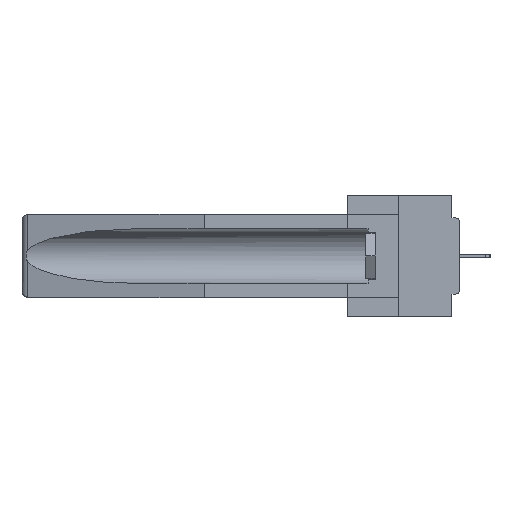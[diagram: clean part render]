
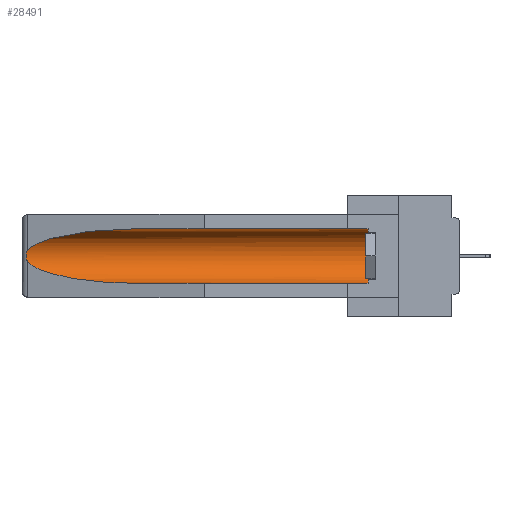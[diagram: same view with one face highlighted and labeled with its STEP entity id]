
A CAD part, left-side view. The second image highlights one B-rep face of the part: STEP entity #28491.
In plain terms, the highlighted cylindrical face has radius 2.857 mm (diameter 5.715 mm), a partial arc.
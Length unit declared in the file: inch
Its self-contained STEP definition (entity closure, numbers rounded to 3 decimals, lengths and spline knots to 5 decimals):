
#315 = CARTESIAN_POINT ( 'NONE',  ( 0.21114, 1.30732, -0.284 ) ) ;
#481 = LINE ( 'NONE', #18571, #19615 ) ;
#2081 = EDGE_CURVE ( 'NONE', #23746, #17120, #19596, .T. ) ;
#2356 = CARTESIAN_POINT ( 'NONE',  ( 0.26655, 1.53094, -0.18657 ) ) ;
#3650 = CARTESIAN_POINT ( 'NONE',  ( 0.155, 0.126, -0.059 ) ) ;
#4187 = ORIENTED_EDGE ( 'NONE', *, *, #26181, .T. ) ;
#4363 = CARTESIAN_POINT ( 'NONE',  ( 0.155, -0.30754, -0.059 ) ) ;
#4367 = LINE ( 'NONE', #4363, #23364 ) ;
#4866 = CARTESIAN_POINT ( 'NONE',  ( 0.26537, 1.52718, -0.19328 ) ) ;
#6810 = VERTEX_POINT ( 'NONE', #25696 ) ;
#7518 = CYLINDRICAL_SURFACE ( 'NONE', #13110, 0.1125 ) ;
#7524 = CARTESIAN_POINT ( 'NONE',  ( 0.155, 0.126, -0.1715 ) ) ;
#8186 = EDGE_CURVE ( 'NONE', #17120, #6810, #4367, .T. ) ;
#8830 = EDGE_CURVE ( 'NONE', #16722, #25071, #17514, .T. ) ;
#9365 = ORIENTED_EDGE ( 'NONE', *, *, #26984, .T. ) ;
#10338 = CARTESIAN_POINT ( 'NONE',  ( 0.26537, 1.52718, -0.19328 ) ) ;
#10518 = EDGE_CURVE ( 'NONE', #23746, #29125, #481, .T. ) ;
#10918 = ORIENTED_EDGE ( 'NONE', *, *, #10518, .F. ) ;
#11493 = CARTESIAN_POINT ( 'NONE',  ( 0.155, 1.07973, -0.059 ) ) ;
#12375 = CARTESIAN_POINT ( 'NONE',  ( 0.26537, 1.52718, -0.14972 ) ) ;
#13110 = AXIS2_PLACEMENT_3D ( 'NONE', #22780, #17799, #20341 ) ;
#13578 = DIRECTION ( 'NONE',  ( 0., 1., 0. ) ) ;
#13954 = CARTESIAN_POINT ( 'NONE',  ( 0.21114, 1.30732, -0.059 ) ) ;
#14334 = DIRECTION ( 'NONE',  ( 0., 1., 0. ) ) ;
#14829 = CARTESIAN_POINT ( 'NONE',  ( 0.2675, 1.53308, -0.16763 ) ) ;
#14921 = FACE_OUTER_BOUND ( 'NONE', #31670, .T. ) ;
#15785 = CARTESIAN_POINT ( 'NONE',  ( 0.26537, 1.52718, -0.19328 ) ) ;
#16444 = CARTESIAN_POINT ( 'NONE',  ( 0.26537, 1.52718, -0.14972 ) ) ;
#16722 = VERTEX_POINT ( 'NONE', #31481 ) ;
#17120 = VERTEX_POINT ( 'NONE', #3650 ) ;
#17335 = CARTESIAN_POINT ( 'NONE',  ( 0.2673, 1.53269, -0.17917 ) ) ;
#17514 = B_SPLINE_CURVE_WITH_KNOTS ( 'NONE', 3,
 ( #12375, #27003, #24555, #29465, #14829, #31859, #17335, #2356, #19803, #4866 ),
 .UNSPECIFIED., .F., .F.,
 ( 4, 2, 2, 2, 4 ),
 ( 0., 0.00029, 0.00058, 0.00087, 0.00117 ),
 .UNSPECIFIED. ) ;
#17539 = DIRECTION ( 'NONE',  ( 0., 0., 1. ) ) ;
#17799 = DIRECTION ( 'NONE',  ( 0., 1., 0. ) ) ;
#17816 = CARTESIAN_POINT ( 'NONE',  ( 0.155, 1.07973, -0.284 ) ) ;
#18571 = CARTESIAN_POINT ( 'NONE',  ( 0.155, -0.30754, -0.284 ) ) ;
#19596 = CIRCLE ( 'NONE', #26715, 0.1125 ) ;
#19615 = VECTOR ( 'NONE', #13578, 39.37008 ) ;
#19803 = CARTESIAN_POINT ( 'NONE',  ( 0.26597, 1.5296, -0.19026 ) ) ;
#20341 = DIRECTION ( 'NONE',  ( 0., 0., 1. ) ) ;
#20509 = CARTESIAN_POINT ( 'NONE',  ( 0.155, 1.07973, -0.284 ) ) ;
#22196 =( BOUNDED_CURVE ( )  B_SPLINE_CURVE ( 3, ( #11493, #13954, #31010, #16444 ),
 .UNSPECIFIED., .F., .F. ) 
 B_SPLINE_CURVE_WITH_KNOTS ( ( 4, 4 ),
 ( 4.71239, 6.08839 ),
 .UNSPECIFIED. ) 
 CURVE ( )  GEOMETRIC_REPRESENTATION_ITEM ( )  RATIONAL_B_SPLINE_CURVE ( ( 1., 0.848, 0.848, 1. ) ) 
 REPRESENTATION_ITEM ( '' )  );
#22448 = ORIENTED_EDGE ( 'NONE', *, *, #8830, .T. ) ;
#22780 = CARTESIAN_POINT ( 'NONE',  ( 0.155, -0.30754, -0.1715 ) ) ;
#23274 = CARTESIAN_POINT ( 'NONE',  ( 0.155, 0.126, -0.284 ) ) ;
#23364 = VECTOR ( 'NONE', #14334, 39.37008 ) ;
#23746 = VERTEX_POINT ( 'NONE', #23274 ) ;
#24555 = CARTESIAN_POINT ( 'NONE',  ( 0.26654, 1.53092, -0.15636 ) ) ;
#24713 = ORIENTED_EDGE ( 'NONE', *, *, #2081, .T. ) ;
#25071 = VERTEX_POINT ( 'NONE', #15785 ) ;
#25117 = DIRECTION ( 'NONE',  ( 0., -1., 0. ) ) ;
#25696 = CARTESIAN_POINT ( 'NONE',  ( 0.155, 1.07973, -0.059 ) ) ;
#26181 = EDGE_CURVE ( 'NONE', #25071, #29125, #31136, .T. ) ;
#26715 = AXIS2_PLACEMENT_3D ( 'NONE', #7524, #25117, #17539 ) ;
#26984 = EDGE_CURVE ( 'NONE', #6810, #16722, #22196, .T. ) ;
#27003 = CARTESIAN_POINT ( 'NONE',  ( 0.26597, 1.52961, -0.15275 ) ) ;
#28491 = ADVANCED_FACE ( 'NONE', ( #14921 ), #7518, .F. ) ;
#29125 = VERTEX_POINT ( 'NONE', #20509 ) ;
#29465 = CARTESIAN_POINT ( 'NONE',  ( 0.2673, 1.5327, -0.16383 ) ) ;
#29907 = CARTESIAN_POINT ( 'NONE',  ( 0.25451, 1.48313, -0.24835 ) ) ;
#31010 = CARTESIAN_POINT ( 'NONE',  ( 0.25451, 1.48313, -0.09465 ) ) ;
#31136 =( BOUNDED_CURVE ( )  B_SPLINE_CURVE ( 3, ( #10338, #29907, #315, #17816 ),
 .UNSPECIFIED., .F., .F. ) 
 B_SPLINE_CURVE_WITH_KNOTS ( ( 4, 4 ),
 ( 0.1948, 1.5708 ),
 .UNSPECIFIED. ) 
 CURVE ( )  GEOMETRIC_REPRESENTATION_ITEM ( )  RATIONAL_B_SPLINE_CURVE ( ( 1., 0.848, 0.848, 1. ) ) 
 REPRESENTATION_ITEM ( '' )  );
#31173 = ORIENTED_EDGE ( 'NONE', *, *, #8186, .T. ) ;
#31481 = CARTESIAN_POINT ( 'NONE',  ( 0.26537, 1.52718, -0.14972 ) ) ;
#31670 = EDGE_LOOP ( 'NONE', ( #9365, #22448, #4187, #10918, #24713, #31173 ) ) ;
#31859 = CARTESIAN_POINT ( 'NONE',  ( 0.2675, 1.53308, -0.17534 ) ) ;
